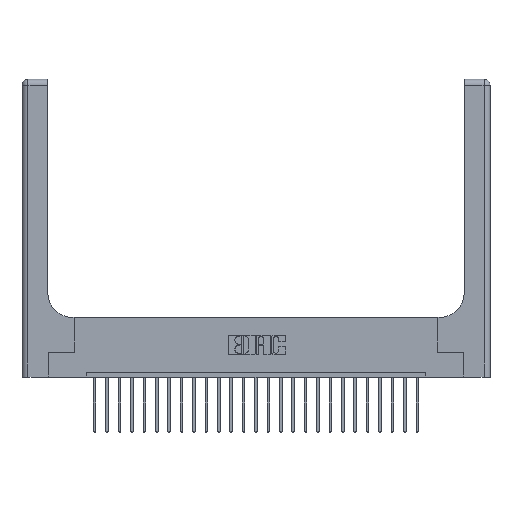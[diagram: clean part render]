
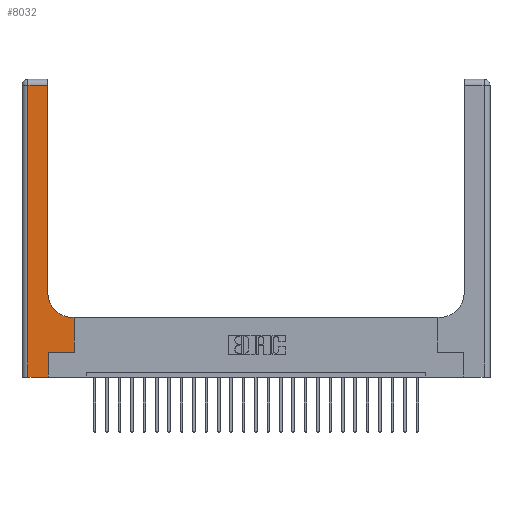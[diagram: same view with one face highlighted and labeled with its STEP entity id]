
A CAD part, top view. The second image highlights one B-rep face of the part: STEP entity #8032.
In plain terms, the highlighted planar face has unit normal (0, 0, 1).
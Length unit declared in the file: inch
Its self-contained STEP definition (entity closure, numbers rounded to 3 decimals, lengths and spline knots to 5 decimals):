
#201 = LINE ( 'NONE', #22326, #20849 ) ;
#237 = CARTESIAN_POINT ( 'NONE',  ( 0.51, 0.85, 0.37 ) ) ;
#419 = VERTEX_POINT ( 'NONE', #9832 ) ;
#474 = DIRECTION ( 'NONE',  ( 0., 0., -1. ) ) ;
#750 = EDGE_CURVE ( 'NONE', #22641, #14514, #16040, .T. ) ;
#1845 = CARTESIAN_POINT ( 'NONE',  ( 0.26, 0.6, 0.37 ) ) ;
#2187 = LINE ( 'NONE', #11571, #3667 ) ;
#2201 = CARTESIAN_POINT ( 'NONE',  ( 0.265, 0., 0.37 ) ) ;
#2488 = CARTESIAN_POINT ( 'NONE',  ( 0.06, 0., 0.37 ) ) ;
#2817 = PLANE ( 'NONE',  #21476 ) ;
#3667 = VECTOR ( 'NONE', #20845, 39.37008 ) ;
#3716 = EDGE_CURVE ( 'NONE', #7436, #19375, #19930, .T. ) ;
#4377 = CARTESIAN_POINT ( 'NONE',  ( 0.265, 0.25, 0.37 ) ) ;
#4622 = CARTESIAN_POINT ( 'NONE',  ( 0.528, 0.25, 0.37 ) ) ;
#4862 = AXIS2_PLACEMENT_3D ( 'NONE', #237, #474, #18879 ) ;
#4915 = VECTOR ( 'NONE', #8864, 39.37008 ) ;
#5287 = CARTESIAN_POINT ( 'NONE',  ( 0.51, 0.6, 0.37 ) ) ;
#5341 = CARTESIAN_POINT ( 'NONE',  ( 0.06, 3., 0.37 ) ) ;
#5388 = CARTESIAN_POINT ( 'NONE',  ( 0.528, 0.25, 0.37 ) ) ;
#5627 = EDGE_CURVE ( 'NONE', #6996, #419, #15491, .T. ) ;
#5968 = CARTESIAN_POINT ( 'NONE',  ( 0., 0., 0.37 ) ) ;
#6392 = VECTOR ( 'NONE', #14378, 39.37008 ) ;
#6534 = DIRECTION ( 'NONE',  ( 0., 0., -1. ) ) ;
#6996 = VERTEX_POINT ( 'NONE', #5287 ) ;
#7059 = VECTOR ( 'NONE', #13498, 39.37008 ) ;
#7119 = EDGE_CURVE ( 'NONE', #10914, #9014, #10965, .T. ) ;
#7436 = VERTEX_POINT ( 'NONE', #5388 ) ;
#8032 = ADVANCED_FACE ( 'NONE', ( #16944 ), #2817, .F. ) ;
#8361 = EDGE_CURVE ( 'NONE', #14514, #23363, #2187, .T. ) ;
#8858 = ORIENTED_EDGE ( 'NONE', *, *, #750, .T. ) ;
#8864 = DIRECTION ( 'NONE',  ( -1., 0., 0. ) ) ;
#9014 = VERTEX_POINT ( 'NONE', #20676 ) ;
#9374 = EDGE_CURVE ( 'NONE', #19375, #6996, #9738, .T. ) ;
#9738 = LINE ( 'NONE', #1845, #17685 ) ;
#9787 = EDGE_CURVE ( 'NONE', #419, #10914, #201, .T. ) ;
#9832 = CARTESIAN_POINT ( 'NONE',  ( 0.26, 0.85, 0.37 ) ) ;
#10168 = ORIENTED_EDGE ( 'NONE', *, *, #9374, .T. ) ;
#10914 = VERTEX_POINT ( 'NONE', #18384 ) ;
#10965 = LINE ( 'NONE', #22088, #4915 ) ;
#11534 = ORIENTED_EDGE ( 'NONE', *, *, #23592, .T. ) ;
#11571 = CARTESIAN_POINT ( 'NONE',  ( 0.265, 0., 0.37 ) ) ;
#11764 = VECTOR ( 'NONE', #21539, 39.37008 ) ;
#12682 = EDGE_CURVE ( 'NONE', #9014, #22641, #20274, .T. ) ;
#13078 = DIRECTION ( 'NONE',  ( -1., 0., 0. ) ) ;
#13175 = DIRECTION ( 'NONE',  ( 0., 1., 0. ) ) ;
#13498 = DIRECTION ( 'NONE',  ( 1., 0., 0. ) ) ;
#13793 = VECTOR ( 'NONE', #14837, 39.37008 ) ;
#13882 = CARTESIAN_POINT ( 'NONE',  ( 0.265, 0.25, 0.37 ) ) ;
#14007 = LINE ( 'NONE', #13882, #11764 ) ;
#14158 = ORIENTED_EDGE ( 'NONE', *, *, #3716, .T. ) ;
#14378 = DIRECTION ( 'NONE',  ( 0., 1., 0. ) ) ;
#14514 = VERTEX_POINT ( 'NONE', #2201 ) ;
#14696 = ORIENTED_EDGE ( 'NONE', *, *, #7119, .T. ) ;
#14837 = DIRECTION ( 'NONE',  ( 0., -1., 0. ) ) ;
#15491 = CIRCLE ( 'NONE', #4862, 0.25 ) ;
#16040 = LINE ( 'NONE', #5968, #7059 ) ;
#16268 = DIRECTION ( 'NONE',  ( -1., 0., 0. ) ) ;
#16371 = ORIENTED_EDGE ( 'NONE', *, *, #9787, .T. ) ;
#16944 = FACE_OUTER_BOUND ( 'NONE', #20339, .T. ) ;
#17685 = VECTOR ( 'NONE', #13078, 39.37008 ) ;
#18384 = CARTESIAN_POINT ( 'NONE',  ( 0.26, 2.94, 0.37 ) ) ;
#18879 = DIRECTION ( 'NONE',  ( 1., 0., 0. ) ) ;
#19375 = VERTEX_POINT ( 'NONE', #21133 ) ;
#19930 = LINE ( 'NONE', #4622, #6392 ) ;
#20274 = LINE ( 'NONE', #5341, #13793 ) ;
#20339 = EDGE_LOOP ( 'NONE', ( #16371, #14696, #22194, #8858, #20975, #11534, #14158, #10168, #23747 ) ) ;
#20676 = CARTESIAN_POINT ( 'NONE',  ( 0.06, 2.94, 0.37 ) ) ;
#20845 = DIRECTION ( 'NONE',  ( 0., 1., 0. ) ) ;
#20849 = VECTOR ( 'NONE', #13175, 39.37008 ) ;
#20975 = ORIENTED_EDGE ( 'NONE', *, *, #8361, .T. ) ;
#21133 = CARTESIAN_POINT ( 'NONE',  ( 0.528, 0.6, 0.37 ) ) ;
#21476 = AXIS2_PLACEMENT_3D ( 'NONE', #23460, #6534, #16268 ) ;
#21539 = DIRECTION ( 'NONE',  ( 1., 0., 0. ) ) ;
#22088 = CARTESIAN_POINT ( 'NONE',  ( 0., 2.94, 0.37 ) ) ;
#22194 = ORIENTED_EDGE ( 'NONE', *, *, #12682, .T. ) ;
#22326 = CARTESIAN_POINT ( 'NONE',  ( 0.26, 3., 0.37 ) ) ;
#22641 = VERTEX_POINT ( 'NONE', #2488 ) ;
#23363 = VERTEX_POINT ( 'NONE', #4377 ) ;
#23460 = CARTESIAN_POINT ( 'NONE',  ( 0., 3., 0.37 ) ) ;
#23592 = EDGE_CURVE ( 'NONE', #23363, #7436, #14007, .T. ) ;
#23747 = ORIENTED_EDGE ( 'NONE', *, *, #5627, .T. ) ;
